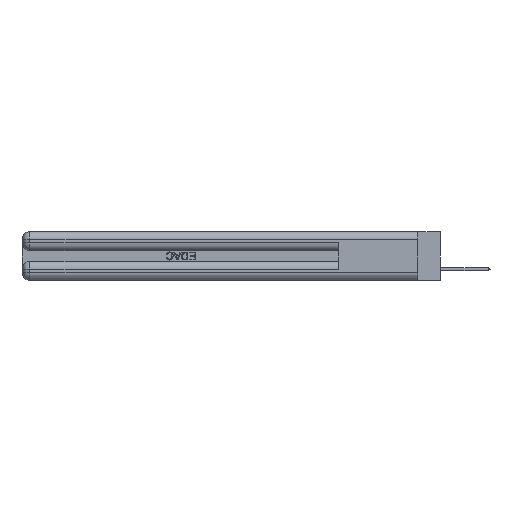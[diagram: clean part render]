
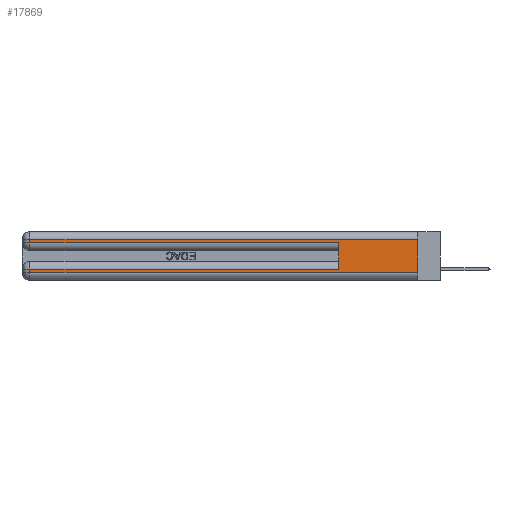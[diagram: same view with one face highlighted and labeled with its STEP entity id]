
A CAD part, left-side view. The second image highlights one B-rep face of the part: STEP entity #17869.
In plain terms, the highlighted planar face has unit normal (-1, 0, 0).
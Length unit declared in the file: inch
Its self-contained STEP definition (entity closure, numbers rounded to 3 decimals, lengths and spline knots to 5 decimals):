
#858 = CARTESIAN_POINT ( 'NONE',  ( 0., 0.6, 0.285 ) ) ;
#1994 = VERTEX_POINT ( 'NONE', #858 ) ;
#2006 = DIRECTION ( 'NONE',  ( 0., 1., 0. ) ) ;
#4017 = LINE ( 'NONE', #24367, #45318 ) ;
#4205 = PLANE ( 'NONE',  #8125 ) ;
#5441 = EDGE_CURVE ( 'NONE', #6165, #36127, #27034, .T. ) ;
#5985 = VECTOR ( 'NONE', #14512, 39.37008 ) ;
#6165 = VERTEX_POINT ( 'NONE', #22656 ) ;
#6331 = EDGE_LOOP ( 'NONE', ( #32416, #7858, #33679, #44505, #43174, #21287, #42514, #37863 ) ) ;
#6721 = LINE ( 'NONE', #23774, #45120 ) ;
#7354 = EDGE_CURVE ( 'NONE', #37099, #41503, #16282, .T. ) ;
#7607 = DIRECTION ( 'NONE',  ( 1., 0., 0. ) ) ;
#7858 = ORIENTED_EDGE ( 'NONE', *, *, #7354, .T. ) ;
#7903 = CARTESIAN_POINT ( 'NONE',  ( 0., 0., 0.37 ) ) ;
#8125 = AXIS2_PLACEMENT_3D ( 'NONE', #7903, #7607, #40917 ) ;
#8662 = EDGE_CURVE ( 'NONE', #27986, #16452, #13311, .T. ) ;
#9164 = EDGE_CURVE ( 'NONE', #16452, #6165, #4017, .T. ) ;
#9873 = VERTEX_POINT ( 'NONE', #24451 ) ;
#12395 = DIRECTION ( 'NONE',  ( 0., 0., 1. ) ) ;
#12766 = VECTOR ( 'NONE', #2006, 39.37008 ) ;
#13311 = LINE ( 'NONE', #15921, #12766 ) ;
#13770 = LINE ( 'NONE', #27096, #47044 ) ;
#13909 = FACE_OUTER_BOUND ( 'NONE', #6331, .T. ) ;
#14197 = CARTESIAN_POINT ( 'NONE',  ( 0., 0., 0.31 ) ) ;
#14439 = DIRECTION ( 'NONE',  ( 0., -1., 0. ) ) ;
#14512 = DIRECTION ( 'NONE',  ( 0., 1., 0. ) ) ;
#15921 = CARTESIAN_POINT ( 'NONE',  ( 0., 0., 0.085 ) ) ;
#16282 = LINE ( 'NONE', #14197, #5985 ) ;
#16452 = VERTEX_POINT ( 'NONE', #41925 ) ;
#17869 = ADVANCED_FACE ( 'NONE', ( #13909 ), #4205, .F. ) ;
#19686 = DIRECTION ( 'NONE',  ( 0., 0., -1. ) ) ;
#20728 = LINE ( 'NONE', #43206, #42543 ) ;
#21250 = VECTOR ( 'NONE', #19686, 39.37008 ) ;
#21287 = ORIENTED_EDGE ( 'NONE', *, *, #8662, .T. ) ;
#21591 = EDGE_CURVE ( 'NONE', #37099, #36127, #20728, .T. ) ;
#22656 = CARTESIAN_POINT ( 'NONE',  ( 0., 2.94, 0.06 ) ) ;
#23774 = CARTESIAN_POINT ( 'NONE',  ( 0., 0.6, 0.145 ) ) ;
#24367 = CARTESIAN_POINT ( 'NONE',  ( 0., 2.94, 0.37 ) ) ;
#24451 = CARTESIAN_POINT ( 'NONE',  ( 0., 2.94, 0.285 ) ) ;
#25005 = CARTESIAN_POINT ( 'NONE',  ( 0., 0., 0.06 ) ) ;
#25175 = CARTESIAN_POINT ( 'NONE',  ( 0., 0.6, 0.085 ) ) ;
#27034 = LINE ( 'NONE', #36395, #32237 ) ;
#27096 = CARTESIAN_POINT ( 'NONE',  ( 0., 0., 0.285 ) ) ;
#27986 = VERTEX_POINT ( 'NONE', #25175 ) ;
#28763 = EDGE_CURVE ( 'NONE', #9873, #1994, #13770, .T. ) ;
#31002 = EDGE_CURVE ( 'NONE', #27986, #1994, #6721, .T. ) ;
#31652 = CARTESIAN_POINT ( 'NONE',  ( 0., 0., 0.31 ) ) ;
#32237 = VECTOR ( 'NONE', #14439, 39.37008 ) ;
#32416 = ORIENTED_EDGE ( 'NONE', *, *, #21591, .F. ) ;
#33295 = CARTESIAN_POINT ( 'NONE',  ( 0., 2.94, 0.31 ) ) ;
#33679 = ORIENTED_EDGE ( 'NONE', *, *, #41145, .T. ) ;
#34429 = CARTESIAN_POINT ( 'NONE',  ( 0., 2.94, 0.37 ) ) ;
#36127 = VERTEX_POINT ( 'NONE', #25005 ) ;
#36395 = CARTESIAN_POINT ( 'NONE',  ( 0., 0., 0.06 ) ) ;
#37099 = VERTEX_POINT ( 'NONE', #31652 ) ;
#37863 = ORIENTED_EDGE ( 'NONE', *, *, #5441, .T. ) ;
#40597 = DIRECTION ( 'NONE',  ( 0., -1., 0. ) ) ;
#40748 = LINE ( 'NONE', #34429, #21250 ) ;
#40917 = DIRECTION ( 'NONE',  ( 0., 0., -1. ) ) ;
#41145 = EDGE_CURVE ( 'NONE', #41503, #9873, #40748, .T. ) ;
#41503 = VERTEX_POINT ( 'NONE', #33295 ) ;
#41925 = CARTESIAN_POINT ( 'NONE',  ( 0., 2.94, 0.085 ) ) ;
#42036 = DIRECTION ( 'NONE',  ( 0., 0., -1. ) ) ;
#42514 = ORIENTED_EDGE ( 'NONE', *, *, #9164, .T. ) ;
#42543 = VECTOR ( 'NONE', #42036, 39.37008 ) ;
#42826 = DIRECTION ( 'NONE',  ( 0., 0., -1. ) ) ;
#43174 = ORIENTED_EDGE ( 'NONE', *, *, #31002, .F. ) ;
#43206 = CARTESIAN_POINT ( 'NONE',  ( 0., 0., 0.37 ) ) ;
#44505 = ORIENTED_EDGE ( 'NONE', *, *, #28763, .T. ) ;
#45120 = VECTOR ( 'NONE', #12395, 39.37008 ) ;
#45318 = VECTOR ( 'NONE', #42826, 39.37008 ) ;
#47044 = VECTOR ( 'NONE', #40597, 39.37008 ) ;
